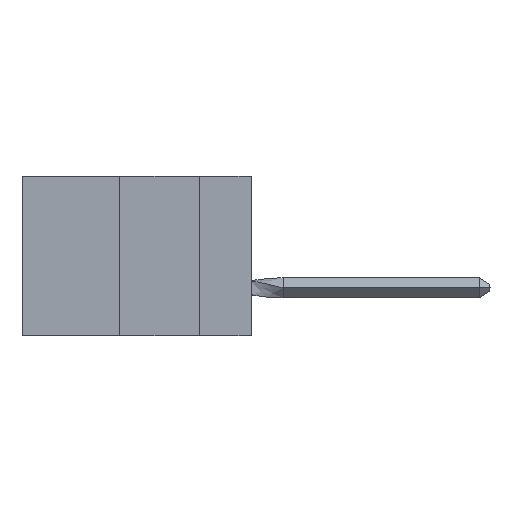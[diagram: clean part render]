
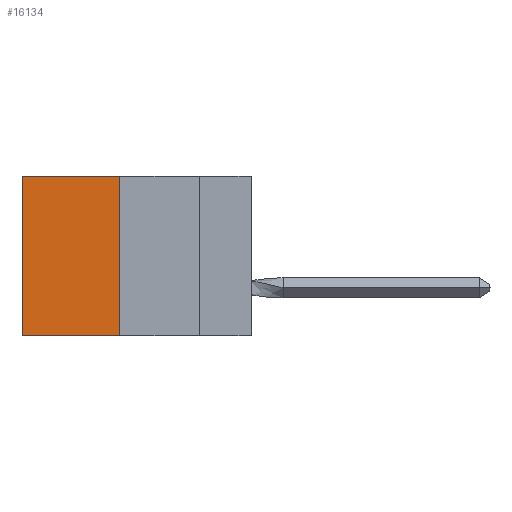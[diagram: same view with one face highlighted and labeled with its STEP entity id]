
A CAD part, left-side view. The second image highlights one B-rep face of the part: STEP entity #16134.
In plain terms, the highlighted planar face has unit normal (-1, 0, 0).
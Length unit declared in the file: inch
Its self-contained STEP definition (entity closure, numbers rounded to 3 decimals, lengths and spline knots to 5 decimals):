
#152 = CARTESIAN_POINT ( 'NONE',  ( 0.305, 0.413, -0.5 ) ) ;
#637 = EDGE_LOOP ( 'NONE', ( #8587, #9154, #8607, #10316 ) ) ;
#652 = CARTESIAN_POINT ( 'NONE',  ( 0.305, 0.413, -0.5 ) ) ;
#1420 = DIRECTION ( 'NONE',  ( 0., 0., -1. ) ) ;
#1625 = LINE ( 'NONE', #6743, #13790 ) ;
#2797 = CARTESIAN_POINT ( 'NONE',  ( 0.305, 0.413, 0. ) ) ;
#3524 = CARTESIAN_POINT ( 'NONE',  ( 0.305, 0.72, 0. ) ) ;
#3683 = DIRECTION ( 'NONE',  ( 0., 0., -1. ) ) ;
#4129 = LINE ( 'NONE', #152, #11809 ) ;
#4784 = DIRECTION ( 'NONE',  ( 1., 0., 0. ) ) ;
#4848 = VECTOR ( 'NONE', #8208, 39.37008 ) ;
#5519 = EDGE_CURVE ( 'NONE', #15139, #10349, #1625, .T. ) ;
#6743 = CARTESIAN_POINT ( 'NONE',  ( 0.305, 0.413, 0. ) ) ;
#7500 = CARTESIAN_POINT ( 'NONE',  ( 0.305, 0.413, -0.5 ) ) ;
#7716 = EDGE_CURVE ( 'NONE', #13378, #9711, #12136, .T. ) ;
#8208 = DIRECTION ( 'NONE',  ( 0., 0., -1. ) ) ;
#8587 = ORIENTED_EDGE ( 'NONE', *, *, #15881, .T. ) ;
#8607 = ORIENTED_EDGE ( 'NONE', *, *, #11098, .F. ) ;
#8781 = FACE_OUTER_BOUND ( 'NONE', #637, .T. ) ;
#8797 = LINE ( 'NONE', #12865, #4848 ) ;
#8805 = CARTESIAN_POINT ( 'NONE',  ( 0.305, 0.413, -0.5 ) ) ;
#9154 = ORIENTED_EDGE ( 'NONE', *, *, #7716, .F. ) ;
#9711 = VERTEX_POINT ( 'NONE', #13350 ) ;
#10316 = ORIENTED_EDGE ( 'NONE', *, *, #5519, .T. ) ;
#10349 = VERTEX_POINT ( 'NONE', #3524 ) ;
#10607 = DIRECTION ( 'NONE',  ( 0., 1., 0. ) ) ;
#11056 = AXIS2_PLACEMENT_3D ( 'NONE', #7500, #4784, #3683 ) ;
#11098 = EDGE_CURVE ( 'NONE', #15139, #13378, #4129, .T. ) ;
#11809 = VECTOR ( 'NONE', #1420, 39.37008 ) ;
#12136 = LINE ( 'NONE', #652, #15848 ) ;
#12865 = CARTESIAN_POINT ( 'NONE',  ( 0.305, 0.72, -0.5 ) ) ;
#13350 = CARTESIAN_POINT ( 'NONE',  ( 0.305, 0.72, -0.5 ) ) ;
#13378 = VERTEX_POINT ( 'NONE', #8805 ) ;
#13620 = PLANE ( 'NONE',  #11056 ) ;
#13790 = VECTOR ( 'NONE', #10607, 39.37008 ) ;
#15139 = VERTEX_POINT ( 'NONE', #2797 ) ;
#15727 = DIRECTION ( 'NONE',  ( 0., 1., 0. ) ) ;
#15848 = VECTOR ( 'NONE', #15727, 39.37008 ) ;
#15881 = EDGE_CURVE ( 'NONE', #10349, #9711, #8797, .T. ) ;
#16134 = ADVANCED_FACE ( 'NONE', ( #8781 ), #13620, .F. ) ;
